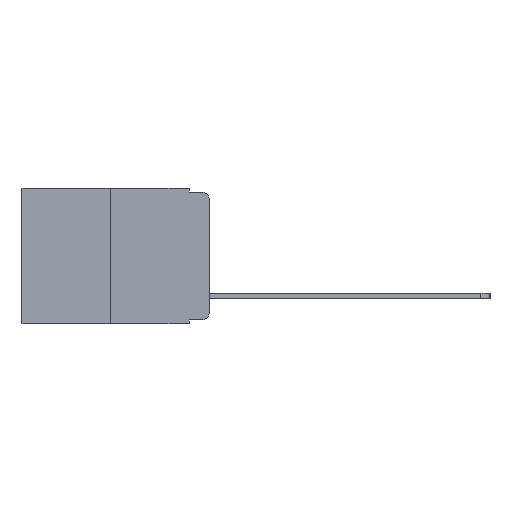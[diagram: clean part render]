
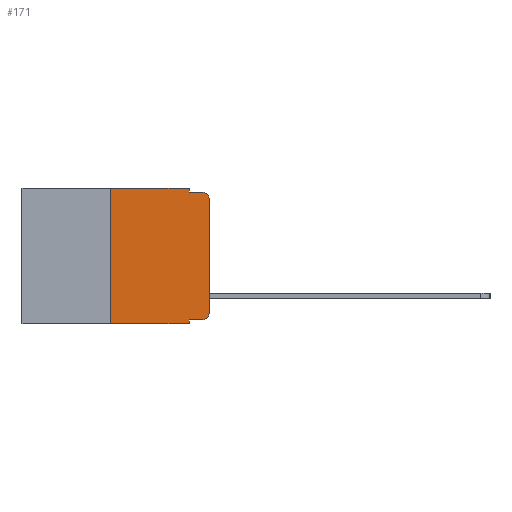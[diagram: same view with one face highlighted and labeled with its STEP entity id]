
A CAD part, left-side view. The second image highlights one B-rep face of the part: STEP entity #171.
In plain terms, the highlighted planar face has unit normal (-1, 0, 0).
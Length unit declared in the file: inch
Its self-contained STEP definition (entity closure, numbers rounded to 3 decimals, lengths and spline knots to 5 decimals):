
#171 = ADVANCED_FACE ( 'NONE', ( #8687 ), #13410, .F. ) ;
#344 = CIRCLE ( 'NONE', #7606, 0.02 ) ;
#393 = VECTOR ( 'NONE', #10046, 39.37008 ) ;
#811 = LINE ( 'NONE', #12134, #393 ) ;
#867 = DIRECTION ( 'NONE',  ( 0., 0., 1. ) ) ;
#976 = VECTOR ( 'NONE', #5338, 39.37008 ) ;
#1032 = AXIS2_PLACEMENT_3D ( 'NONE', #12585, #12487, #12609 ) ;
#1112 = CARTESIAN_POINT ( 'NONE',  ( 0., 0.02, -0.313 ) ) ;
#1255 = VERTEX_POINT ( 'NONE', #3625 ) ;
#1361 = ORIENTED_EDGE ( 'NONE', *, *, #2116, .T. ) ;
#1465 = EDGE_LOOP ( 'NONE', ( #13762, #5692, #11659, #3495, #3843, #6727, #12340, #9891, #1361, #10210 ) ) ;
#1782 = VERTEX_POINT ( 'NONE', #8938 ) ;
#1819 = EDGE_CURVE ( 'NONE', #1255, #3475, #5097, .T. ) ;
#1921 = CARTESIAN_POINT ( 'NONE',  ( 0., 0., -0.313 ) ) ;
#2078 = VECTOR ( 'NONE', #2123, 39.37008 ) ;
#2108 = CARTESIAN_POINT ( 'NONE',  ( 0., 0.02, -0.333 ) ) ;
#2116 = EDGE_CURVE ( 'NONE', #4771, #13904, #7795, .T. ) ;
#2123 = DIRECTION ( 'NONE',  ( 0., -1., 0. ) ) ;
#2322 = VERTEX_POINT ( 'NONE', #4496 ) ;
#2405 = DIRECTION ( 'NONE',  ( 0., 0., -1. ) ) ;
#2839 = CARTESIAN_POINT ( 'NONE',  ( 0., 0.051, -0.343 ) ) ;
#2950 = EDGE_CURVE ( 'NONE', #1782, #1255, #11753, .T. ) ;
#3002 = VERTEX_POINT ( 'NONE', #13073 ) ;
#3441 = CARTESIAN_POINT ( 'NONE',  ( 0., 0.051, -0.333 ) ) ;
#3475 = VERTEX_POINT ( 'NONE', #9655 ) ;
#3495 = ORIENTED_EDGE ( 'NONE', *, *, #13909, .F. ) ;
#3520 = VECTOR ( 'NONE', #9785, 39.37008 ) ;
#3625 = CARTESIAN_POINT ( 'NONE',  ( 0., 0.25, 0. ) ) ;
#3843 = ORIENTED_EDGE ( 'NONE', *, *, #1819, .F. ) ;
#4446 = EDGE_CURVE ( 'NONE', #4771, #13125, #811, .T. ) ;
#4496 = CARTESIAN_POINT ( 'NONE',  ( 0., 0., -0.03 ) ) ;
#4771 = VERTEX_POINT ( 'NONE', #3441 ) ;
#5097 = LINE ( 'NONE', #8802, #2078 ) ;
#5338 = DIRECTION ( 'NONE',  ( 0., 0., 1. ) ) ;
#5363 = LINE ( 'NONE', #5925, #7892 ) ;
#5692 = ORIENTED_EDGE ( 'NONE', *, *, #10433, .T. ) ;
#5925 = CARTESIAN_POINT ( 'NONE',  ( 0., 0.051, -0.01 ) ) ;
#6173 = CARTESIAN_POINT ( 'NONE',  ( 0., 0.02, -0.03 ) ) ;
#6250 = EDGE_CURVE ( 'NONE', #13904, #10585, #10306, .T. ) ;
#6372 = VECTOR ( 'NONE', #8005, 39.37008 ) ;
#6410 = LINE ( 'NONE', #8722, #3520 ) ;
#6727 = ORIENTED_EDGE ( 'NONE', *, *, #2950, .F. ) ;
#7124 = VECTOR ( 'NONE', #12289, 39.37008 ) ;
#7246 = DIRECTION ( 'NONE',  ( 0., 0., -1. ) ) ;
#7606 = AXIS2_PLACEMENT_3D ( 'NONE', #6173, #13530, #7246 ) ;
#7725 = LINE ( 'NONE', #9619, #976 ) ;
#7795 = LINE ( 'NONE', #13088, #7124 ) ;
#7892 = VECTOR ( 'NONE', #13304, 39.37008 ) ;
#8005 = DIRECTION ( 'NONE',  ( 0., -1., 0. ) ) ;
#8687 = FACE_OUTER_BOUND ( 'NONE', #1465, .T. ) ;
#8722 = CARTESIAN_POINT ( 'NONE',  ( 0., 0.051, 0. ) ) ;
#8802 = CARTESIAN_POINT ( 'NONE',  ( 0., 0.473, 0. ) ) ;
#8938 = CARTESIAN_POINT ( 'NONE',  ( 0., 0.25, -0.343 ) ) ;
#8980 = VECTOR ( 'NONE', #867, 39.37008 ) ;
#8984 = DIRECTION ( 'NONE',  ( -1., 0., 0. ) ) ;
#9049 = EDGE_CURVE ( 'NONE', #10650, #3002, #5363, .T. ) ;
#9308 = EDGE_CURVE ( 'NONE', #10585, #2322, #7725, .T. ) ;
#9619 = CARTESIAN_POINT ( 'NONE',  ( 0., 0., 0. ) ) ;
#9655 = CARTESIAN_POINT ( 'NONE',  ( 0., 0.051, 0. ) ) ;
#9720 = CARTESIAN_POINT ( 'NONE',  ( 0., 0.051, -0.01 ) ) ;
#9785 = DIRECTION ( 'NONE',  ( 0., 0., -1. ) ) ;
#9891 = ORIENTED_EDGE ( 'NONE', *, *, #4446, .F. ) ;
#10046 = DIRECTION ( 'NONE',  ( 0., 0., -1. ) ) ;
#10210 = ORIENTED_EDGE ( 'NONE', *, *, #6250, .T. ) ;
#10260 = EDGE_CURVE ( 'NONE', #1782, #13125, #12652, .T. ) ;
#10306 = CIRCLE ( 'NONE', #14120, 0.02 ) ;
#10433 = EDGE_CURVE ( 'NONE', #2322, #3002, #344, .T. ) ;
#10585 = VERTEX_POINT ( 'NONE', #1921 ) ;
#10650 = VERTEX_POINT ( 'NONE', #9720 ) ;
#11158 = CARTESIAN_POINT ( 'NONE',  ( 0., 0.473, -0.343 ) ) ;
#11659 = ORIENTED_EDGE ( 'NONE', *, *, #9049, .F. ) ;
#11753 = LINE ( 'NONE', #14074, #8980 ) ;
#12134 = CARTESIAN_POINT ( 'NONE',  ( 0., 0.051, 0. ) ) ;
#12289 = DIRECTION ( 'NONE',  ( 0., -1., 0. ) ) ;
#12340 = ORIENTED_EDGE ( 'NONE', *, *, #10260, .T. ) ;
#12487 = DIRECTION ( 'NONE',  ( 1., 0., 0. ) ) ;
#12585 = CARTESIAN_POINT ( 'NONE',  ( 0., 0.473, 0. ) ) ;
#12609 = DIRECTION ( 'NONE',  ( 0., 0., -1. ) ) ;
#12652 = LINE ( 'NONE', #11158, #6372 ) ;
#13073 = CARTESIAN_POINT ( 'NONE',  ( 0., 0.02, -0.01 ) ) ;
#13088 = CARTESIAN_POINT ( 'NONE',  ( 0., 0.051, -0.333 ) ) ;
#13125 = VERTEX_POINT ( 'NONE', #2839 ) ;
#13304 = DIRECTION ( 'NONE',  ( 0., -1., 0. ) ) ;
#13410 = PLANE ( 'NONE',  #1032 ) ;
#13530 = DIRECTION ( 'NONE',  ( -1., 0., 0. ) ) ;
#13762 = ORIENTED_EDGE ( 'NONE', *, *, #9308, .T. ) ;
#13904 = VERTEX_POINT ( 'NONE', #2108 ) ;
#13909 = EDGE_CURVE ( 'NONE', #3475, #10650, #6410, .T. ) ;
#14074 = CARTESIAN_POINT ( 'NONE',  ( 0., 0.25, 0. ) ) ;
#14120 = AXIS2_PLACEMENT_3D ( 'NONE', #1112, #8984, #2405 ) ;
